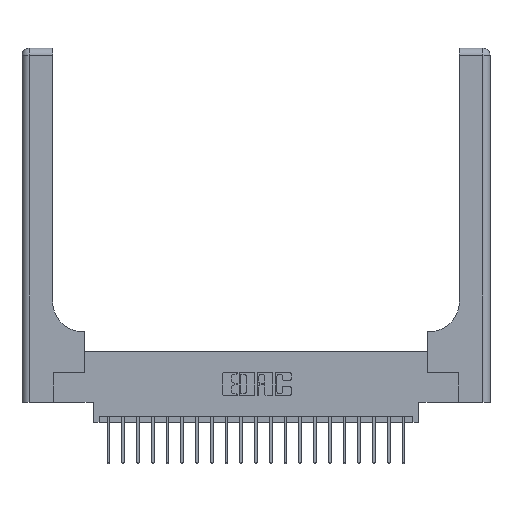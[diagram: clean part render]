
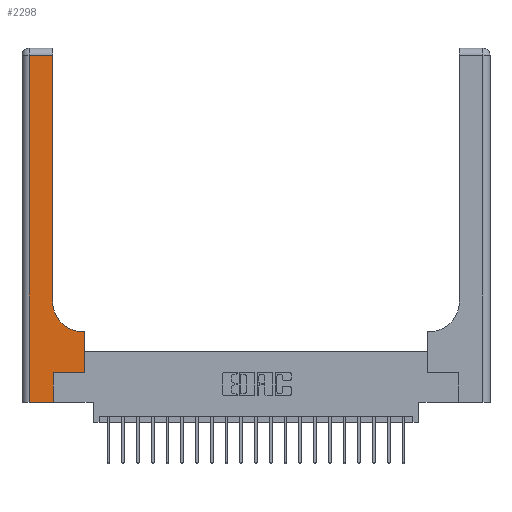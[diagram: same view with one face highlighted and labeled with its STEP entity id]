
A CAD part, top view. The second image highlights one B-rep face of the part: STEP entity #2298.
In plain terms, the highlighted planar face has unit normal (0, 0, 1).
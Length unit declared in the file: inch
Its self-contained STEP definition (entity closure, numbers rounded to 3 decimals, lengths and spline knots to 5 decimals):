
#329 = ORIENTED_EDGE ( 'NONE', *, *, #1861, .T. ) ;
#705 = VECTOR ( 'NONE', #8601, 39.37008 ) ;
#1053 = VECTOR ( 'NONE', #16520, 39.37008 ) ;
#1221 = EDGE_CURVE ( 'NONE', #16678, #9783, #14386, .T. ) ;
#1228 = CARTESIAN_POINT ( 'NONE',  ( 0.265, 0.25, 0.37 ) ) ;
#1861 = EDGE_CURVE ( 'NONE', #21137, #16678, #6240, .T. ) ;
#2130 = CIRCLE ( 'NONE', #9691, 0.25 ) ;
#2211 = CARTESIAN_POINT ( 'NONE',  ( 0.528, 0.25, 0.37 ) ) ;
#2298 = ADVANCED_FACE ( 'NONE', ( #19712 ), #5937, .F. ) ;
#2462 = VECTOR ( 'NONE', #16286, 39.37008 ) ;
#2690 = CARTESIAN_POINT ( 'NONE',  ( 0.265, 0., 0.37 ) ) ;
#3275 = CARTESIAN_POINT ( 'NONE',  ( 0., 0., 0.37 ) ) ;
#3344 = VECTOR ( 'NONE', #12493, 39.37008 ) ;
#3606 = VERTEX_POINT ( 'NONE', #21201 ) ;
#4431 = EDGE_CURVE ( 'NONE', #13787, #5566, #2130, .T. ) ;
#4515 = EDGE_CURVE ( 'NONE', #5656, #21137, #11867, .T. ) ;
#4650 = CARTESIAN_POINT ( 'NONE',  ( 0.51, 0.85, 0.37 ) ) ;
#5155 = EDGE_LOOP ( 'NONE', ( #17916, #7978, #7173, #9491, #329, #17270, #6271, #19616, #15322 ) ) ;
#5566 = VERTEX_POINT ( 'NONE', #19997 ) ;
#5656 = VERTEX_POINT ( 'NONE', #8142 ) ;
#5710 = CARTESIAN_POINT ( 'NONE',  ( 0.265, 0.25, 0.37 ) ) ;
#5937 = PLANE ( 'NONE',  #8624 ) ;
#6240 = LINE ( 'NONE', #19897, #2462 ) ;
#6271 = ORIENTED_EDGE ( 'NONE', *, *, #12955, .T. ) ;
#6385 = DIRECTION ( 'NONE',  ( 0., 0., -1. ) ) ;
#6547 = EDGE_CURVE ( 'NONE', #3606, #13787, #7531, .T. ) ;
#6709 = VECTOR ( 'NONE', #16087, 39.37008 ) ;
#7173 = ORIENTED_EDGE ( 'NONE', *, *, #12838, .T. ) ;
#7300 = CARTESIAN_POINT ( 'NONE',  ( 0.26, 0.6, 0.37 ) ) ;
#7416 = LINE ( 'NONE', #19490, #3344 ) ;
#7531 = LINE ( 'NONE', #7300, #17803 ) ;
#7812 = DIRECTION ( 'NONE',  ( 1., 0., 0. ) ) ;
#7978 = ORIENTED_EDGE ( 'NONE', *, *, #18154, .T. ) ;
#8004 = VERTEX_POINT ( 'NONE', #21423 ) ;
#8142 = CARTESIAN_POINT ( 'NONE',  ( 0.06, 0., 0.37 ) ) ;
#8601 = DIRECTION ( 'NONE',  ( 1., 0., 0. ) ) ;
#8624 = AXIS2_PLACEMENT_3D ( 'NONE', #18010, #6385, #18456 ) ;
#9241 = EDGE_CURVE ( 'NONE', #5566, #16037, #19412, .T. ) ;
#9491 = ORIENTED_EDGE ( 'NONE', *, *, #4515, .T. ) ;
#9691 = AXIS2_PLACEMENT_3D ( 'NONE', #4650, #11531, #7812 ) ;
#9783 = VERTEX_POINT ( 'NONE', #2211 ) ;
#10634 = CARTESIAN_POINT ( 'NONE',  ( 0.528, 0.25, 0.37 ) ) ;
#11531 = DIRECTION ( 'NONE',  ( 0., 0., -1. ) ) ;
#11867 = LINE ( 'NONE', #3275, #705 ) ;
#12216 = DIRECTION ( 'NONE',  ( 0., 1., 0. ) ) ;
#12272 = CARTESIAN_POINT ( 'NONE',  ( 0.51, 0.6, 0.37 ) ) ;
#12493 = DIRECTION ( 'NONE',  ( -1., 0., 0. ) ) ;
#12838 = EDGE_CURVE ( 'NONE', #8004, #5656, #20023, .T. ) ;
#12955 = EDGE_CURVE ( 'NONE', #9783, #3606, #17520, .T. ) ;
#13348 = CARTESIAN_POINT ( 'NONE',  ( 0.26, 2.94, 0.37 ) ) ;
#13787 = VERTEX_POINT ( 'NONE', #12272 ) ;
#13983 = CARTESIAN_POINT ( 'NONE',  ( 0.26, 3., 0.37 ) ) ;
#14386 = LINE ( 'NONE', #5710, #6709 ) ;
#15322 = ORIENTED_EDGE ( 'NONE', *, *, #4431, .T. ) ;
#16037 = VERTEX_POINT ( 'NONE', #13348 ) ;
#16087 = DIRECTION ( 'NONE',  ( 1., 0., 0. ) ) ;
#16286 = DIRECTION ( 'NONE',  ( 0., 1., 0. ) ) ;
#16520 = DIRECTION ( 'NONE',  ( 0., -1., 0. ) ) ;
#16678 = VERTEX_POINT ( 'NONE', #1228 ) ;
#17270 = ORIENTED_EDGE ( 'NONE', *, *, #1221, .T. ) ;
#17520 = LINE ( 'NONE', #10634, #21974 ) ;
#17803 = VECTOR ( 'NONE', #18011, 39.37008 ) ;
#17916 = ORIENTED_EDGE ( 'NONE', *, *, #9241, .T. ) ;
#18010 = CARTESIAN_POINT ( 'NONE',  ( 0., 3., 0.37 ) ) ;
#18011 = DIRECTION ( 'NONE',  ( -1., 0., 0. ) ) ;
#18154 = EDGE_CURVE ( 'NONE', #16037, #8004, #7416, .T. ) ;
#18416 = VECTOR ( 'NONE', #20897, 39.37008 ) ;
#18456 = DIRECTION ( 'NONE',  ( -1., 0., 0. ) ) ;
#19412 = LINE ( 'NONE', #13983, #18416 ) ;
#19490 = CARTESIAN_POINT ( 'NONE',  ( 0., 2.94, 0.37 ) ) ;
#19616 = ORIENTED_EDGE ( 'NONE', *, *, #6547, .T. ) ;
#19712 = FACE_OUTER_BOUND ( 'NONE', #5155, .T. ) ;
#19897 = CARTESIAN_POINT ( 'NONE',  ( 0.265, 0., 0.37 ) ) ;
#19997 = CARTESIAN_POINT ( 'NONE',  ( 0.26, 0.85, 0.37 ) ) ;
#20023 = LINE ( 'NONE', #22061, #1053 ) ;
#20897 = DIRECTION ( 'NONE',  ( 0., 1., 0. ) ) ;
#21137 = VERTEX_POINT ( 'NONE', #2690 ) ;
#21201 = CARTESIAN_POINT ( 'NONE',  ( 0.528, 0.6, 0.37 ) ) ;
#21423 = CARTESIAN_POINT ( 'NONE',  ( 0.06, 2.94, 0.37 ) ) ;
#21974 = VECTOR ( 'NONE', #12216, 39.37008 ) ;
#22061 = CARTESIAN_POINT ( 'NONE',  ( 0.06, 3., 0.37 ) ) ;
